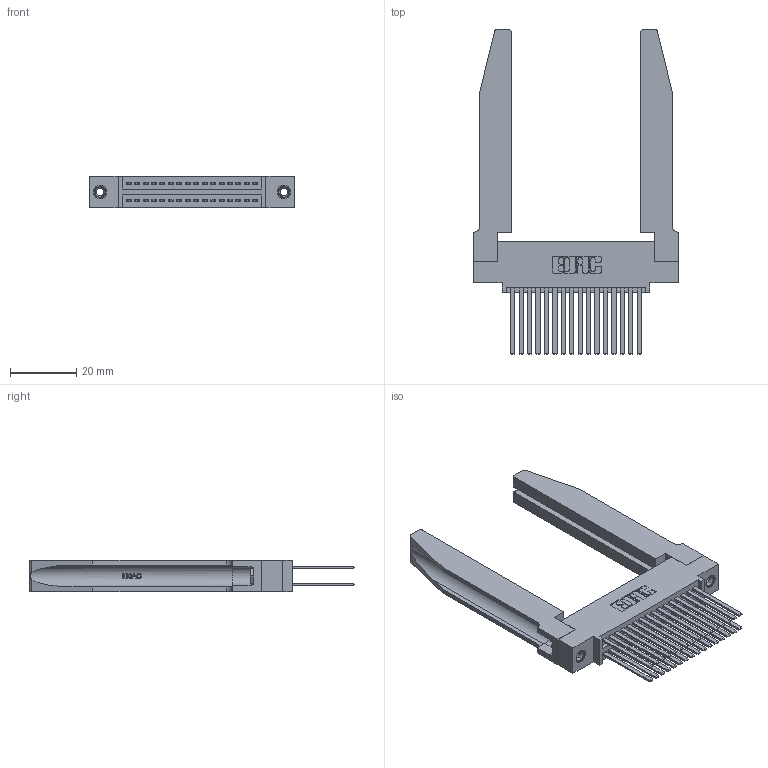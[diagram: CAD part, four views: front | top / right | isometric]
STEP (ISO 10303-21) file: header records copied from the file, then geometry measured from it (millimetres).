
FILE_DESCRIPTION (( 'STEP AP203' ), '1' );
FILE_NAME ('345-032-544-578.STEP', '2019-10-28T04:38:23', ( '' ), ( '' ), 'SwSTEP 2.0', 'SolidWorks 2016', '' );
FILE_SCHEMA (( 'CONFIG_CONTROL_DESIGN' ));
Length unit declared in the file: inch
Products named in the file (5): 345-292-001_345-293-144; 345-032-544-578; 345-250-001_345-250-001-102; 345 Part_0.110 Offset - 0.156 Dia-TH; 345-220-078_345-220-078
Assembly tree (37 placements, depth 2):
  345-032-544-578
    345 Part_0.110 Offset - 0.156 Dia-TH
    345-292-001_345-293-144  x32
    345-250-001_345-250-001-102  x2
    345-220-078_345-220-078  x2
Bounding box: 61.87 x 97.71 x 9.4 mm (x, y, z)
Volume: 13914.8 mm3; surface area: 16825 mm2
Topology: 37 solids, 37 shells, 1772 faces, 5153 edges, 3382 vertices
Faces by surface type: plane 1154, cylinder 566, bspline 36, cone 12, torus 4
Entity records: 20742 total; most frequent: CARTESIAN_POINT 4419, ORIENTED_EDGE 3250, DIRECTION 2919, EDGE_CURVE 1625, VECTOR 1339, LINE 1339, VERTEX_POINT 1076, AXIS2_PLACEMENT_3D 790
